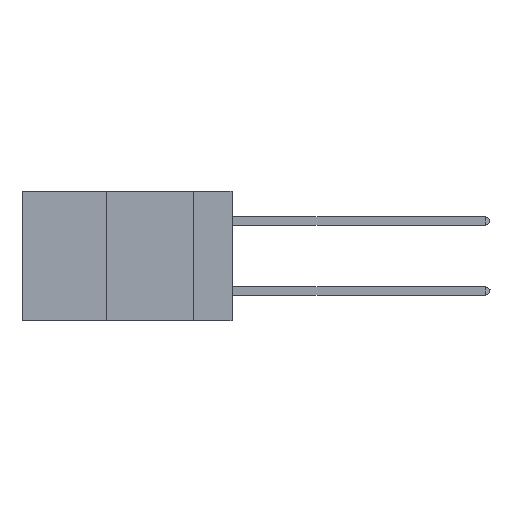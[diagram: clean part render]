
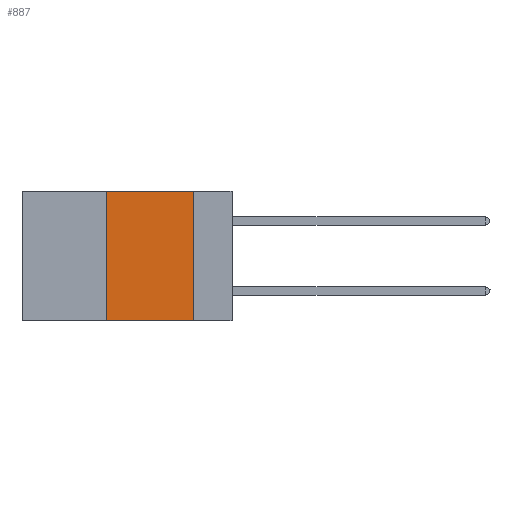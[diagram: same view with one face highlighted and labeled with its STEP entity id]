
A CAD part, left-side view. The second image highlights one B-rep face of the part: STEP entity #887.
In plain terms, the highlighted planar face has unit normal (-1, 0, 0).
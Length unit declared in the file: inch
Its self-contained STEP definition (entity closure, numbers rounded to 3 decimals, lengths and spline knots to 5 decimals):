
#641 = ORIENTED_EDGE ( 'NONE', *, *, #16260, .F. ) ;
#887 = ADVANCED_FACE ( 'NONE', ( #15788 ), #27023, .F. ) ;
#2612 = DIRECTION ( 'NONE',  ( 0., 0., -1. ) ) ;
#4989 = CARTESIAN_POINT ( 'NONE',  ( 0., 0.36, 0. ) ) ;
#5009 = ORIENTED_EDGE ( 'NONE', *, *, #26303, .F. ) ;
#5609 = VERTEX_POINT ( 'NONE', #17347 ) ;
#6002 = ORIENTED_EDGE ( 'NONE', *, *, #17905, .T. ) ;
#6440 = CARTESIAN_POINT ( 'NONE',  ( 0., 0.36, 0. ) ) ;
#6480 = CARTESIAN_POINT ( 'NONE',  ( 0., 0.6, 0. ) ) ;
#6630 = DIRECTION ( 'NONE',  ( 0., 0., -1. ) ) ;
#7466 = VERTEX_POINT ( 'NONE', #4989 ) ;
#10663 = EDGE_LOOP ( 'NONE', ( #641, #5009, #26201, #6002 ) ) ;
#10714 = VECTOR ( 'NONE', #2612, 39.37008 ) ;
#11191 = LINE ( 'NONE', #18381, #10714 ) ;
#11271 = EDGE_CURVE ( 'NONE', #17662, #7466, #26982, .T. ) ;
#12294 = VECTOR ( 'NONE', #18838, 39.37008 ) ;
#12579 = CARTESIAN_POINT ( 'NONE',  ( 0., 0.6, 0. ) ) ;
#13493 = DIRECTION ( 'NONE',  ( 0., 0., 1. ) ) ;
#13611 = CARTESIAN_POINT ( 'NONE',  ( 0., 0.36, -0.37 ) ) ;
#14481 = LINE ( 'NONE', #23192, #12294 ) ;
#15627 = DIRECTION ( 'NONE',  ( 1., 0., 0. ) ) ;
#15788 = FACE_OUTER_BOUND ( 'NONE', #10663, .T. ) ;
#16260 = EDGE_CURVE ( 'NONE', #29180, #5609, #11191, .T. ) ;
#17347 = CARTESIAN_POINT ( 'NONE',  ( 0., 0.11, -0.37 ) ) ;
#17662 = VERTEX_POINT ( 'NONE', #13611 ) ;
#17905 = EDGE_CURVE ( 'NONE', #17662, #5609, #14481, .T. ) ;
#18381 = CARTESIAN_POINT ( 'NONE',  ( 0., 0.11, 0. ) ) ;
#18838 = DIRECTION ( 'NONE',  ( 0., -1., 0. ) ) ;
#19324 = DIRECTION ( 'NONE',  ( 0., -1., 0. ) ) ;
#20999 = LINE ( 'NONE', #12579, #22066 ) ;
#22066 = VECTOR ( 'NONE', #19324, 39.37008 ) ;
#23189 = AXIS2_PLACEMENT_3D ( 'NONE', #6480, #15627, #6630 ) ;
#23192 = CARTESIAN_POINT ( 'NONE',  ( 0., 0.6, -0.37 ) ) ;
#26201 = ORIENTED_EDGE ( 'NONE', *, *, #11271, .F. ) ;
#26303 = EDGE_CURVE ( 'NONE', #7466, #29180, #20999, .T. ) ;
#26982 = LINE ( 'NONE', #6440, #29588 ) ;
#27023 = PLANE ( 'NONE',  #23189 ) ;
#27723 = CARTESIAN_POINT ( 'NONE',  ( 0., 0.11, 0. ) ) ;
#29180 = VERTEX_POINT ( 'NONE', #27723 ) ;
#29588 = VECTOR ( 'NONE', #13493, 39.37008 ) ;
